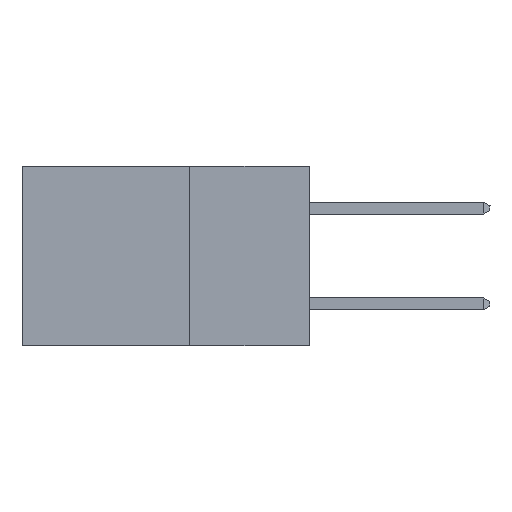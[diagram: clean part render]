
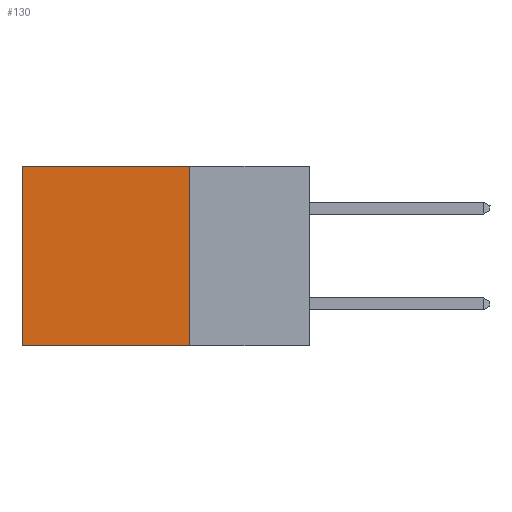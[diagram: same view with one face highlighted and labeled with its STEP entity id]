
A CAD part, left-side view. The second image highlights one B-rep face of the part: STEP entity #130.
In plain terms, the highlighted planar face has unit normal (-1, 0, 0).
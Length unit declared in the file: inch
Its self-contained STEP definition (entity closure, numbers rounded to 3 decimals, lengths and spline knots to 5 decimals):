
#130 = ADVANCED_FACE ( 'NONE', ( #1811 ), #8303, .F. ) ;
#1042 = VECTOR ( 'NONE', #2415, 39.37008 ) ;
#1447 = AXIS2_PLACEMENT_3D ( 'NONE', #2984, #3882, #3058 ) ;
#1767 = CARTESIAN_POINT ( 'NONE',  ( 0.2875, 0.25, -0.375 ) ) ;
#1811 = FACE_OUTER_BOUND ( 'NONE', #6473, .T. ) ;
#1841 = ORIENTED_EDGE ( 'NONE', *, *, #3173, .F. ) ;
#2133 = VECTOR ( 'NONE', #8136, 39.37008 ) ;
#2415 = DIRECTION ( 'NONE',  ( 0., 0., -1. ) ) ;
#2545 = LINE ( 'NONE', #12055, #2133 ) ;
#2984 = CARTESIAN_POINT ( 'NONE',  ( 0.2875, 0.25, -0.375 ) ) ;
#3058 = DIRECTION ( 'NONE',  ( 0., 0., -1. ) ) ;
#3173 = EDGE_CURVE ( 'NONE', #8768, #9194, #2545, .T. ) ;
#3882 = DIRECTION ( 'NONE',  ( 1., 0., 0. ) ) ;
#4253 = CARTESIAN_POINT ( 'NONE',  ( 0.2875, 0.25, 0. ) ) ;
#4394 = LINE ( 'NONE', #4253, #9871 ) ;
#6094 = ORIENTED_EDGE ( 'NONE', *, *, #6191, .T. ) ;
#6191 = EDGE_CURVE ( 'NONE', #11627, #12549, #9883, .T. ) ;
#6473 = EDGE_LOOP ( 'NONE', ( #6094, #13150, #1841, #6635 ) ) ;
#6635 = ORIENTED_EDGE ( 'NONE', *, *, #8000, .T. ) ;
#7627 = CARTESIAN_POINT ( 'NONE',  ( 0.2875, 0.6, 0. ) ) ;
#8000 = EDGE_CURVE ( 'NONE', #8768, #11627, #4394, .T. ) ;
#8136 = DIRECTION ( 'NONE',  ( 0., 0., -1. ) ) ;
#8303 = PLANE ( 'NONE',  #1447 ) ;
#8425 = CARTESIAN_POINT ( 'NONE',  ( 0.2875, 0.25, 0. ) ) ;
#8768 = VERTEX_POINT ( 'NONE', #8425 ) ;
#9194 = VERTEX_POINT ( 'NONE', #1767 ) ;
#9201 = DIRECTION ( 'NONE',  ( 0., 1., 0. ) ) ;
#9520 = DIRECTION ( 'NONE',  ( 0., 1., 0. ) ) ;
#9688 = VECTOR ( 'NONE', #9201, 39.37008 ) ;
#9871 = VECTOR ( 'NONE', #9520, 39.37008 ) ;
#9883 = LINE ( 'NONE', #12115, #1042 ) ;
#11627 = VERTEX_POINT ( 'NONE', #7627 ) ;
#12055 = CARTESIAN_POINT ( 'NONE',  ( 0.2875, 0.25, -0.375 ) ) ;
#12115 = CARTESIAN_POINT ( 'NONE',  ( 0.2875, 0.6, -0.375 ) ) ;
#12540 = CARTESIAN_POINT ( 'NONE',  ( 0.2875, 0.25, -0.375 ) ) ;
#12549 = VERTEX_POINT ( 'NONE', #13424 ) ;
#13150 = ORIENTED_EDGE ( 'NONE', *, *, #13393, .F. ) ;
#13393 = EDGE_CURVE ( 'NONE', #9194, #12549, #13582, .T. ) ;
#13424 = CARTESIAN_POINT ( 'NONE',  ( 0.2875, 0.6, -0.375 ) ) ;
#13582 = LINE ( 'NONE', #12540, #9688 ) ;
